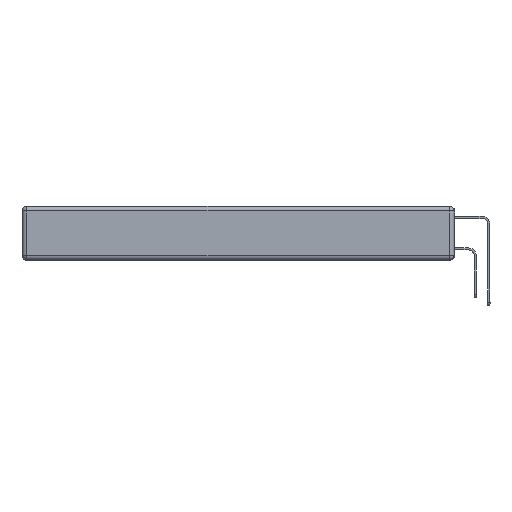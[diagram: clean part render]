
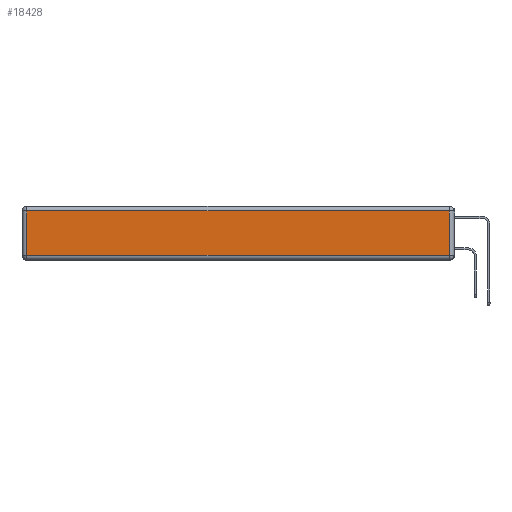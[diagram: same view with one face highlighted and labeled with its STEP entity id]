
A CAD part, left-side view. The second image highlights one B-rep face of the part: STEP entity #18428.
In plain terms, the highlighted planar face has unit normal (-1, 0, 0).
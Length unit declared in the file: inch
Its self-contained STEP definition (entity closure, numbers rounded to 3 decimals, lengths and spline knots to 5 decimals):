
#211 = DIRECTION ( 'NONE',  ( 0., 0., -1. ) ) ;
#339 = CARTESIAN_POINT ( 'NONE',  ( 0., 2.75, -0.03 ) ) ;
#978 = VERTEX_POINT ( 'NONE', #3644 ) ;
#2396 = LINE ( 'NONE', #21545, #6911 ) ;
#2476 = ORIENTED_EDGE ( 'NONE', *, *, #24218, .T. ) ;
#3644 = CARTESIAN_POINT ( 'NONE',  ( 0., 2.72, -0.03 ) ) ;
#4783 = CARTESIAN_POINT ( 'NONE',  ( 0., 2.72, -0.313 ) ) ;
#5706 = CARTESIAN_POINT ( 'NONE',  ( 0., 0.03, -0.313 ) ) ;
#6355 = FACE_OUTER_BOUND ( 'NONE', #18203, .T. ) ;
#6911 = VECTOR ( 'NONE', #10023, 39.37008 ) ;
#6933 = AXIS2_PLACEMENT_3D ( 'NONE', #19763, #10246, #8365 ) ;
#6964 = VERTEX_POINT ( 'NONE', #11562 ) ;
#7587 = DIRECTION ( 'NONE',  ( 0., 1., 0. ) ) ;
#7930 = VECTOR ( 'NONE', #211, 39.37008 ) ;
#7936 = EDGE_CURVE ( 'NONE', #16074, #22994, #9740, .T. ) ;
#8365 = DIRECTION ( 'NONE',  ( 0., 0., 1. ) ) ;
#8791 = VECTOR ( 'NONE', #23388, 39.37008 ) ;
#9204 = ORIENTED_EDGE ( 'NONE', *, *, #11056, .T. ) ;
#9740 = LINE ( 'NONE', #17375, #8791 ) ;
#9836 = LINE ( 'NONE', #339, #13892 ) ;
#10023 = DIRECTION ( 'NONE',  ( 0., 0., 1. ) ) ;
#10246 = DIRECTION ( 'NONE',  ( -1., 0., 0. ) ) ;
#11056 = EDGE_CURVE ( 'NONE', #22994, #6964, #2396, .T. ) ;
#11347 = CARTESIAN_POINT ( 'NONE',  ( 0., 2.72, -0.343 ) ) ;
#11562 = CARTESIAN_POINT ( 'NONE',  ( 0., 0.03, -0.03 ) ) ;
#12118 = PLANE ( 'NONE',  #6933 ) ;
#13870 = ORIENTED_EDGE ( 'NONE', *, *, #7936, .T. ) ;
#13892 = VECTOR ( 'NONE', #7587, 39.37008 ) ;
#16074 = VERTEX_POINT ( 'NONE', #4783 ) ;
#17375 = CARTESIAN_POINT ( 'NONE',  ( 0., 0., -0.313 ) ) ;
#18203 = EDGE_LOOP ( 'NONE', ( #13870, #9204, #2476, #23619 ) ) ;
#18428 = ADVANCED_FACE ( 'NONE', ( #6355 ), #12118, .T. ) ;
#19099 = LINE ( 'NONE', #11347, #7930 ) ;
#19763 = CARTESIAN_POINT ( 'NONE',  ( 0., 0., -0.343 ) ) ;
#21545 = CARTESIAN_POINT ( 'NONE',  ( 0., 0.03, -0.343 ) ) ;
#22959 = EDGE_CURVE ( 'NONE', #978, #16074, #19099, .T. ) ;
#22994 = VERTEX_POINT ( 'NONE', #5706 ) ;
#23388 = DIRECTION ( 'NONE',  ( 0., -1., 0. ) ) ;
#23619 = ORIENTED_EDGE ( 'NONE', *, *, #22959, .T. ) ;
#24218 = EDGE_CURVE ( 'NONE', #6964, #978, #9836, .T. ) ;
